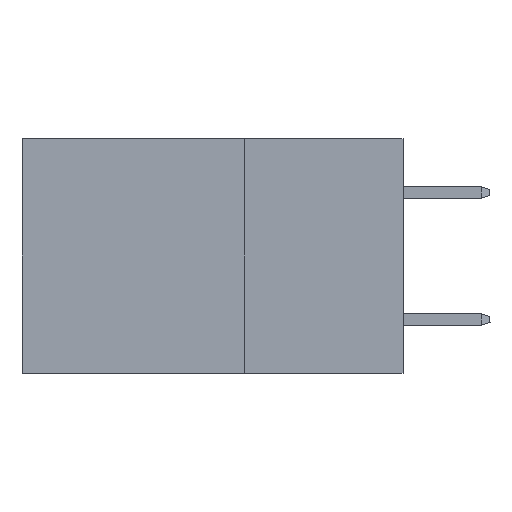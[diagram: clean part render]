
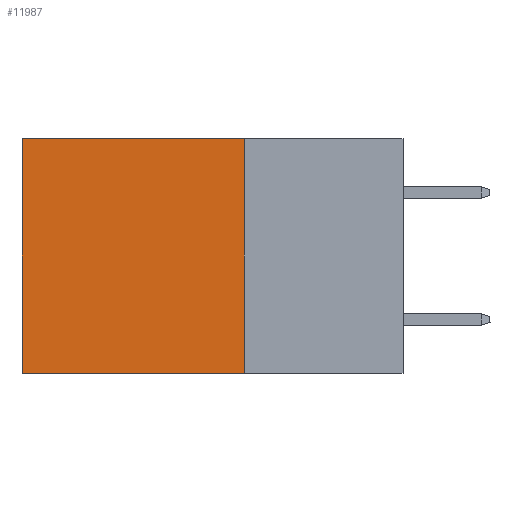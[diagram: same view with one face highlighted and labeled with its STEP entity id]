
A CAD part, left-side view. The second image highlights one B-rep face of the part: STEP entity #11987.
In plain terms, the highlighted planar face has unit normal (-1, 0, 0).
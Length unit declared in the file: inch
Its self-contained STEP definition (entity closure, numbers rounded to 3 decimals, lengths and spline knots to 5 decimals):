
#27 = DIRECTION ( 'NONE',  ( 0., 0., -1. ) ) ;
#924 = CARTESIAN_POINT ( 'NONE',  ( 0.2875, 0.6, -0.37 ) ) ;
#3015 = CARTESIAN_POINT ( 'NONE',  ( 0.2875, 0.25, -0.37 ) ) ;
#3163 = CARTESIAN_POINT ( 'NONE',  ( 0.2875, 0.25, 0. ) ) ;
#3513 = FACE_OUTER_BOUND ( 'NONE', #9838, .T. ) ;
#3630 = CARTESIAN_POINT ( 'NONE',  ( 0.2875, 0.25, 0. ) ) ;
#5234 = ORIENTED_EDGE ( 'NONE', *, *, #18080, .F. ) ;
#5532 = DIRECTION ( 'NONE',  ( 0., 0., -1. ) ) ;
#5607 = CARTESIAN_POINT ( 'NONE',  ( 0.2875, 0.25, 0. ) ) ;
#5839 = EDGE_CURVE ( 'NONE', #14431, #10874, #21051, .T. ) ;
#6737 = DIRECTION ( 'NONE',  ( 0., 1., 0. ) ) ;
#7473 = CARTESIAN_POINT ( 'NONE',  ( 0.2875, 0.25, 0. ) ) ;
#8222 = ORIENTED_EDGE ( 'NONE', *, *, #10514, .F. ) ;
#8811 = CARTESIAN_POINT ( 'NONE',  ( 0.2875, 0.6, 0. ) ) ;
#9838 = EDGE_LOOP ( 'NONE', ( #11685, #5234, #8222, #19259 ) ) ;
#10514 = EDGE_CURVE ( 'NONE', #15421, #15015, #13305, .T. ) ;
#10874 = VERTEX_POINT ( 'NONE', #924 ) ;
#11685 = ORIENTED_EDGE ( 'NONE', *, *, #5839, .T. ) ;
#11987 = ADVANCED_FACE ( 'NONE', ( #3513 ), #19094, .F. ) ;
#12103 = VECTOR ( 'NONE', #6737, 39.37008 ) ;
#12817 = DIRECTION ( 'NONE',  ( 0., 1., 0. ) ) ;
#13072 = LINE ( 'NONE', #3015, #24023 ) ;
#13230 = DIRECTION ( 'NONE',  ( 0., 0., -1. ) ) ;
#13305 = LINE ( 'NONE', #3630, #15705 ) ;
#13538 = CARTESIAN_POINT ( 'NONE',  ( 0.2875, 0.25, -0.37 ) ) ;
#14431 = VERTEX_POINT ( 'NONE', #24856 ) ;
#14514 = LINE ( 'NONE', #3163, #12103 ) ;
#15015 = VERTEX_POINT ( 'NONE', #13538 ) ;
#15421 = VERTEX_POINT ( 'NONE', #5607 ) ;
#15705 = VECTOR ( 'NONE', #27, 39.37008 ) ;
#16370 = EDGE_CURVE ( 'NONE', #15421, #14431, #14514, .T. ) ;
#17191 = VECTOR ( 'NONE', #13230, 39.37008 ) ;
#18080 = EDGE_CURVE ( 'NONE', #15015, #10874, #13072, .T. ) ;
#19094 = PLANE ( 'NONE',  #23425 ) ;
#19259 = ORIENTED_EDGE ( 'NONE', *, *, #16370, .T. ) ;
#21051 = LINE ( 'NONE', #8811, #17191 ) ;
#23052 = DIRECTION ( 'NONE',  ( 1., 0., 0. ) ) ;
#23425 = AXIS2_PLACEMENT_3D ( 'NONE', #7473, #23052, #5532 ) ;
#24023 = VECTOR ( 'NONE', #12817, 39.37008 ) ;
#24856 = CARTESIAN_POINT ( 'NONE',  ( 0.2875, 0.6, 0. ) ) ;
